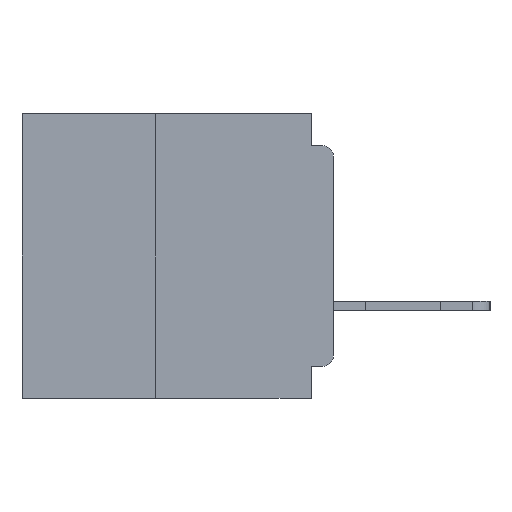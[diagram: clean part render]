
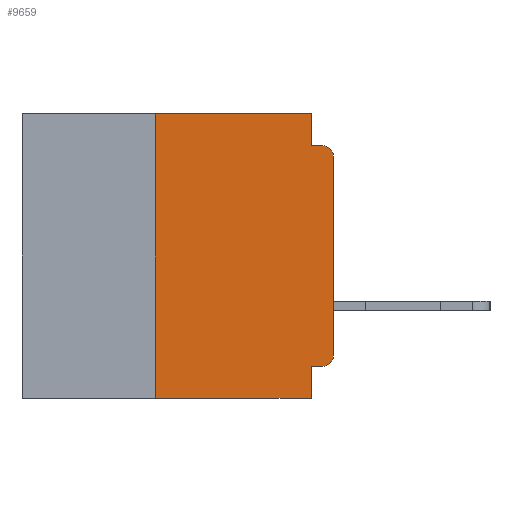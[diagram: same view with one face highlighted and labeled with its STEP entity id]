
A CAD part, left-side view. The second image highlights one B-rep face of the part: STEP entity #9659.
In plain terms, the highlighted planar face has unit normal (-1, 0, 0).
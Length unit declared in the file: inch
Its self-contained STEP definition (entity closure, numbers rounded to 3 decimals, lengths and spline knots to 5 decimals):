
#28 = DIRECTION ( 'NONE',  ( 0., 0., -1. ) ) ;
#377 = LINE ( 'NONE', #2171, #30021 ) ;
#732 = VERTEX_POINT ( 'NONE', #12304 ) ;
#885 = EDGE_CURVE ( 'NONE', #1821, #30575, #8907, .T. ) ;
#1821 = VERTEX_POINT ( 'NONE', #29940 ) ;
#1902 = ORIENTED_EDGE ( 'NONE', *, *, #31040, .F. ) ;
#2107 = LINE ( 'NONE', #11359, #31739 ) ;
#2171 = CARTESIAN_POINT ( 'NONE',  ( 0., 0.031, -0.4 ) ) ;
#2177 = CARTESIAN_POINT ( 'NONE',  ( 0., 0.031, -0.4 ) ) ;
#4132 = AXIS2_PLACEMENT_3D ( 'NONE', #34281, #17216, #28 ) ;
#4454 = CARTESIAN_POINT ( 'NONE',  ( 0., 0.031, -0.045 ) ) ;
#5063 = CARTESIAN_POINT ( 'NONE',  ( 0., 0.437, 0. ) ) ;
#5378 = CIRCLE ( 'NONE', #18668, 0.015 ) ;
#6544 = CARTESIAN_POINT ( 'NONE',  ( 0., 0., -0.045 ) ) ;
#6706 = VERTEX_POINT ( 'NONE', #11501 ) ;
#7686 = ORIENTED_EDGE ( 'NONE', *, *, #25695, .T. ) ;
#7746 = VECTOR ( 'NONE', #25247, 39.37008 ) ;
#7771 = VECTOR ( 'NONE', #35956, 39.37008 ) ;
#7775 = CARTESIAN_POINT ( 'NONE',  ( 0., 0.015, -0.355 ) ) ;
#7851 = ORIENTED_EDGE ( 'NONE', *, *, #885, .F. ) ;
#8651 = LINE ( 'NONE', #33214, #7771 ) ;
#8907 = LINE ( 'NONE', #18520, #23331 ) ;
#9659 = ADVANCED_FACE ( 'NONE', ( #31675 ), #33908, .F. ) ;
#10245 = EDGE_CURVE ( 'NONE', #732, #1821, #12735, .T. ) ;
#10409 = LINE ( 'NONE', #26958, #24850 ) ;
#11266 = DIRECTION ( 'NONE',  ( -1., 0., 0. ) ) ;
#11278 = EDGE_CURVE ( 'NONE', #16510, #13029, #8651, .T. ) ;
#11359 = CARTESIAN_POINT ( 'NONE',  ( 0., 0., 0. ) ) ;
#11501 = CARTESIAN_POINT ( 'NONE',  ( 0., 0., -0.34 ) ) ;
#12304 = CARTESIAN_POINT ( 'NONE',  ( 0., 0.25, 0. ) ) ;
#12735 = LINE ( 'NONE', #5063, #20420 ) ;
#12945 = VECTOR ( 'NONE', #26677, 39.37008 ) ;
#13029 = VERTEX_POINT ( 'NONE', #2177 ) ;
#14788 = EDGE_LOOP ( 'NONE', ( #7686, #28739, #1902, #7851, #15991, #16538, #23995, #33909, #27755, #30563 ) ) ;
#15392 = DIRECTION ( 'NONE',  ( 0., 1., 0. ) ) ;
#15576 = VERTEX_POINT ( 'NONE', #7775 ) ;
#15991 = ORIENTED_EDGE ( 'NONE', *, *, #10245, .F. ) ;
#16510 = VERTEX_POINT ( 'NONE', #34855 ) ;
#16538 = ORIENTED_EDGE ( 'NONE', *, *, #28603, .F. ) ;
#16826 = DIRECTION ( 'NONE',  ( 1., 0., 0. ) ) ;
#17043 = AXIS2_PLACEMENT_3D ( 'NONE', #31132, #16826, #36649 ) ;
#17137 = DIRECTION ( 'NONE',  ( 0., 0., -1. ) ) ;
#17216 = DIRECTION ( 'NONE',  ( -1., 0., 0. ) ) ;
#17361 = DIRECTION ( 'NONE',  ( 0., 0., -1. ) ) ;
#17903 = CARTESIAN_POINT ( 'NONE',  ( 0., 0.031, -0.355 ) ) ;
#18520 = CARTESIAN_POINT ( 'NONE',  ( 0., 0.031, 0. ) ) ;
#18668 = AXIS2_PLACEMENT_3D ( 'NONE', #28535, #11266, #31407 ) ;
#19718 = LINE ( 'NONE', #6544, #12945 ) ;
#20420 = VECTOR ( 'NONE', #25195, 39.37008 ) ;
#21920 = EDGE_CURVE ( 'NONE', #15576, #27602, #10409, .T. ) ;
#22361 = CARTESIAN_POINT ( 'NONE',  ( 0., 0.25, -0.4 ) ) ;
#22508 = CARTESIAN_POINT ( 'NONE',  ( 0., 0.015, -0.045 ) ) ;
#22919 = EDGE_CURVE ( 'NONE', #31848, #31884, #28814, .T. ) ;
#22951 = DIRECTION ( 'NONE',  ( 0., 0., 1. ) ) ;
#23059 = LINE ( 'NONE', #22361, #7746 ) ;
#23331 = VECTOR ( 'NONE', #17361, 39.37008 ) ;
#23995 = ORIENTED_EDGE ( 'NONE', *, *, #11278, .T. ) ;
#24850 = VECTOR ( 'NONE', #15392, 39.37008 ) ;
#25195 = DIRECTION ( 'NONE',  ( 0., -1., 0. ) ) ;
#25247 = DIRECTION ( 'NONE',  ( 0., 0., 1. ) ) ;
#25695 = EDGE_CURVE ( 'NONE', #6706, #31848, #2107, .T. ) ;
#26677 = DIRECTION ( 'NONE',  ( 0., -1., 0. ) ) ;
#26958 = CARTESIAN_POINT ( 'NONE',  ( 0., 0., -0.355 ) ) ;
#27602 = VERTEX_POINT ( 'NONE', #17903 ) ;
#27755 = ORIENTED_EDGE ( 'NONE', *, *, #21920, .F. ) ;
#28535 = CARTESIAN_POINT ( 'NONE',  ( 0., 0.015, -0.34 ) ) ;
#28603 = EDGE_CURVE ( 'NONE', #16510, #732, #23059, .T. ) ;
#28739 = ORIENTED_EDGE ( 'NONE', *, *, #22919, .T. ) ;
#28814 = CIRCLE ( 'NONE', #4132, 0.015 ) ;
#29940 = CARTESIAN_POINT ( 'NONE',  ( 0., 0.031, 0. ) ) ;
#30021 = VECTOR ( 'NONE', #17137, 39.37008 ) ;
#30563 = ORIENTED_EDGE ( 'NONE', *, *, #33772, .T. ) ;
#30575 = VERTEX_POINT ( 'NONE', #4454 ) ;
#31040 = EDGE_CURVE ( 'NONE', #30575, #31884, #19718, .T. ) ;
#31132 = CARTESIAN_POINT ( 'NONE',  ( 0., 0.437, 0. ) ) ;
#31338 = EDGE_CURVE ( 'NONE', #27602, #13029, #377, .T. ) ;
#31407 = DIRECTION ( 'NONE',  ( 0., 0., -1. ) ) ;
#31675 = FACE_OUTER_BOUND ( 'NONE', #14788, .T. ) ;
#31739 = VECTOR ( 'NONE', #22951, 39.37008 ) ;
#31848 = VERTEX_POINT ( 'NONE', #36559 ) ;
#31884 = VERTEX_POINT ( 'NONE', #22508 ) ;
#33214 = CARTESIAN_POINT ( 'NONE',  ( 0., 0.437, -0.4 ) ) ;
#33772 = EDGE_CURVE ( 'NONE', #15576, #6706, #5378, .T. ) ;
#33908 = PLANE ( 'NONE',  #17043 ) ;
#33909 = ORIENTED_EDGE ( 'NONE', *, *, #31338, .F. ) ;
#34281 = CARTESIAN_POINT ( 'NONE',  ( 0., 0.015, -0.06 ) ) ;
#34855 = CARTESIAN_POINT ( 'NONE',  ( 0., 0.25, -0.4 ) ) ;
#35956 = DIRECTION ( 'NONE',  ( 0., -1., 0. ) ) ;
#36559 = CARTESIAN_POINT ( 'NONE',  ( 0., 0., -0.06 ) ) ;
#36649 = DIRECTION ( 'NONE',  ( 0., 0., -1. ) ) ;
